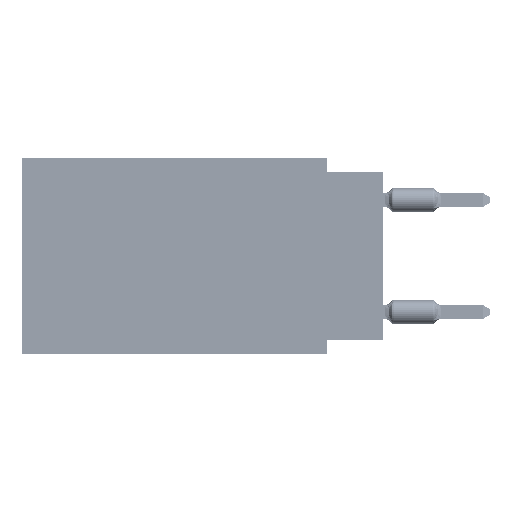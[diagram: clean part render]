
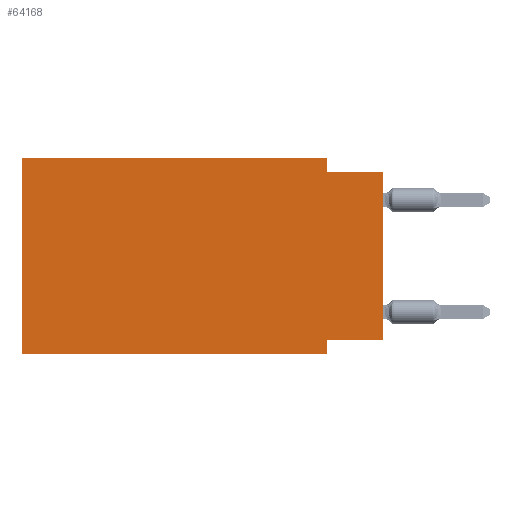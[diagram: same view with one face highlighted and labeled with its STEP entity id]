
A CAD part, left-side view. The second image highlights one B-rep face of the part: STEP entity #64168.
In plain terms, the highlighted planar face has unit normal (-1, 0, 0).
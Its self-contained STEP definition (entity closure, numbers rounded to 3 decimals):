
#860 = CARTESIAN_POINT ( 'NONE',  ( 0., 16.383, 0. ) ) ;
#2038 = ORIENTED_EDGE ( 'NONE', *, *, #16194, .F. ) ;
#2632 = CARTESIAN_POINT ( 'NONE',  ( 0., 2.54, 0. ) ) ;
#5664 = EDGE_CURVE ( 'NONE', #64211, #68939, #17394, .T. ) ;
#6156 = CARTESIAN_POINT ( 'NONE',  ( 0., 2.54, -0.635 ) ) ;
#8725 = DIRECTION ( 'NONE',  ( 0., -1., 0. ) ) ;
#9001 = CARTESIAN_POINT ( 'NONE',  ( 0., 16.383, 0. ) ) ;
#11225 = ORIENTED_EDGE ( 'NONE', *, *, #54833, .F. ) ;
#11935 = VERTEX_POINT ( 'NONE', #65549 ) ;
#11984 = LINE ( 'NONE', #77762, #58464 ) ;
#14285 = LINE ( 'NONE', #29978, #18682 ) ;
#14491 = ORIENTED_EDGE ( 'NONE', *, *, #89865, .F. ) ;
#16194 = EDGE_CURVE ( 'NONE', #68939, #63415, #89580, .T. ) ;
#17394 = LINE ( 'NONE', #2632, #55923 ) ;
#17640 = EDGE_CURVE ( 'NONE', #29105, #63415, #11984, .T. ) ;
#18403 = CARTESIAN_POINT ( 'NONE',  ( 0., 16.383, -8.89 ) ) ;
#18682 = VECTOR ( 'NONE', #37333, 1000. ) ;
#18830 = DIRECTION ( 'NONE',  ( 0., 0., -1. ) ) ;
#19435 = VECTOR ( 'NONE', #8725, 1000. ) ;
#20554 = EDGE_CURVE ( 'NONE', #68485, #11935, #55139, .T. ) ;
#22823 = EDGE_CURVE ( 'NONE', #68485, #72659, #60533, .T. ) ;
#29105 = VERTEX_POINT ( 'NONE', #47520 ) ;
#29978 = CARTESIAN_POINT ( 'NONE',  ( 0., 2.54, -8.89 ) ) ;
#32568 = CARTESIAN_POINT ( 'NONE',  ( 0., 16.383, -8.89 ) ) ;
#37333 = DIRECTION ( 'NONE',  ( 0., 0., -1. ) ) ;
#38943 = DIRECTION ( 'NONE',  ( 0., 0., 1. ) ) ;
#39435 = VECTOR ( 'NONE', #43950, 1000. ) ;
#40660 = EDGE_LOOP ( 'NONE', ( #61721, #2038, #83033, #94584, #73484, #54531, #11225, #14491 ) ) ;
#41521 = VECTOR ( 'NONE', #80915, 1000. ) ;
#43950 = DIRECTION ( 'NONE',  ( 0., -1., 0. ) ) ;
#45905 = DIRECTION ( 'NONE',  ( 0., 0., -1. ) ) ;
#46486 = AXIS2_PLACEMENT_3D ( 'NONE', #51830, #53763, #45905 ) ;
#46869 = VERTEX_POINT ( 'NONE', #93454 ) ;
#47103 = CARTESIAN_POINT ( 'NONE',  ( 0., 0., -0.635 ) ) ;
#47520 = CARTESIAN_POINT ( 'NONE',  ( 0., 0., -8.255 ) ) ;
#49756 = DIRECTION ( 'NONE',  ( 0., 0., 1. ) ) ;
#51830 = CARTESIAN_POINT ( 'NONE',  ( 0., 16.383, 0. ) ) ;
#53763 = DIRECTION ( 'NONE',  ( 1., 0., 0. ) ) ;
#54531 = ORIENTED_EDGE ( 'NONE', *, *, #20554, .T. ) ;
#54833 = EDGE_CURVE ( 'NONE', #46869, #11935, #14285, .T. ) ;
#55139 = LINE ( 'NONE', #32568, #87021 ) ;
#55610 = DIRECTION ( 'NONE',  ( 0., -1., 0. ) ) ;
#55923 = VECTOR ( 'NONE', #18830, 1000. ) ;
#58188 = CARTESIAN_POINT ( 'NONE',  ( 0., 0., -0.635 ) ) ;
#58464 = VECTOR ( 'NONE', #49756, 1000. ) ;
#60436 = EDGE_CURVE ( 'NONE', #72659, #64211, #83818, .T. ) ;
#60533 = LINE ( 'NONE', #9001, #84211 ) ;
#60764 = CARTESIAN_POINT ( 'NONE',  ( 0., 0., -8.255 ) ) ;
#61721 = ORIENTED_EDGE ( 'NONE', *, *, #17640, .T. ) ;
#63415 = VERTEX_POINT ( 'NONE', #47103 ) ;
#64168 = ADVANCED_FACE ( 'NONE', ( #67035 ), #75858, .F. ) ;
#64211 = VERTEX_POINT ( 'NONE', #83707 ) ;
#65549 = CARTESIAN_POINT ( 'NONE',  ( 0., 2.54, -8.89 ) ) ;
#67035 = FACE_OUTER_BOUND ( 'NONE', #40660, .T. ) ;
#68063 = CARTESIAN_POINT ( 'NONE',  ( 0., 16.383, 0. ) ) ;
#68485 = VERTEX_POINT ( 'NONE', #18403 ) ;
#68939 = VERTEX_POINT ( 'NONE', #6156 ) ;
#72659 = VERTEX_POINT ( 'NONE', #68063 ) ;
#73484 = ORIENTED_EDGE ( 'NONE', *, *, #22823, .F. ) ;
#75009 = LINE ( 'NONE', #60764, #41521 ) ;
#75858 = PLANE ( 'NONE',  #46486 ) ;
#77762 = CARTESIAN_POINT ( 'NONE',  ( 0., 0., 0. ) ) ;
#80915 = DIRECTION ( 'NONE',  ( 0., 1., 0. ) ) ;
#83033 = ORIENTED_EDGE ( 'NONE', *, *, #5664, .F. ) ;
#83707 = CARTESIAN_POINT ( 'NONE',  ( 0., 2.54, 0. ) ) ;
#83818 = LINE ( 'NONE', #860, #19435 ) ;
#84211 = VECTOR ( 'NONE', #38943, 1000. ) ;
#87021 = VECTOR ( 'NONE', #55610, 1000. ) ;
#89580 = LINE ( 'NONE', #58188, #39435 ) ;
#89865 = EDGE_CURVE ( 'NONE', #29105, #46869, #75009, .T. ) ;
#93454 = CARTESIAN_POINT ( 'NONE',  ( 0., 2.54, -8.255 ) ) ;
#94584 = ORIENTED_EDGE ( 'NONE', *, *, #60436, .F. ) ;
